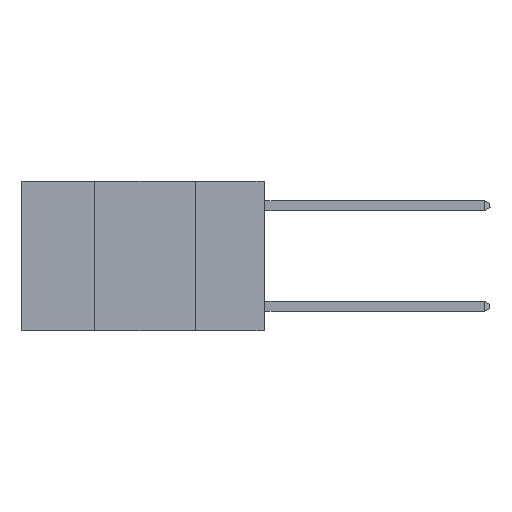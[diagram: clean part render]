
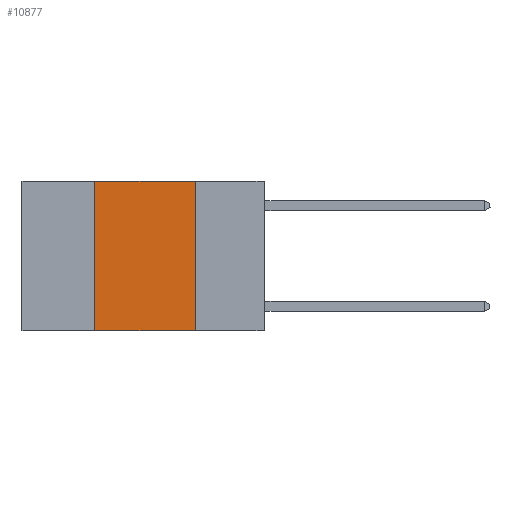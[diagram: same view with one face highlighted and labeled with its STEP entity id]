
A CAD part, left-side view. The second image highlights one B-rep face of the part: STEP entity #10877.
In plain terms, the highlighted planar face has unit normal (-1, 0, 0).
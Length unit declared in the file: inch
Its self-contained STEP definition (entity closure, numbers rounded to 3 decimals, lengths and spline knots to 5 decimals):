
#200 = AXIS2_PLACEMENT_3D ( 'NONE', #25338, #23256, #19574 ) ;
#3056 = CARTESIAN_POINT ( 'NONE',  ( 0., 0.17, 0. ) ) ;
#4137 = VECTOR ( 'NONE', #25794, 39.37008 ) ;
#4219 = CARTESIAN_POINT ( 'NONE',  ( 0., 0.6, 0. ) ) ;
#5190 = CARTESIAN_POINT ( 'NONE',  ( 0., 0.6, -0.37 ) ) ;
#5335 = LINE ( 'NONE', #5190, #27424 ) ;
#6482 = VERTEX_POINT ( 'NONE', #24693 ) ;
#6800 = CARTESIAN_POINT ( 'NONE',  ( 0., 0.42, 0. ) ) ;
#9617 = CARTESIAN_POINT ( 'NONE',  ( 0., 0.17, -0.37 ) ) ;
#9890 = EDGE_CURVE ( 'NONE', #15368, #20033, #17591, .T. ) ;
#10433 = DIRECTION ( 'NONE',  ( 0., 0., 1. ) ) ;
#10745 = EDGE_CURVE ( 'NONE', #6482, #15368, #25072, .T. ) ;
#10877 = ADVANCED_FACE ( 'NONE', ( #12530 ), #21025, .F. ) ;
#11447 = CARTESIAN_POINT ( 'NONE',  ( 0., 0.17, 0. ) ) ;
#12530 = FACE_OUTER_BOUND ( 'NONE', #26441, .T. ) ;
#12691 = VECTOR ( 'NONE', #10433, 39.37008 ) ;
#13400 = VERTEX_POINT ( 'NONE', #9617 ) ;
#14685 = ORIENTED_EDGE ( 'NONE', *, *, #10745, .F. ) ;
#15368 = VERTEX_POINT ( 'NONE', #6800 ) ;
#16486 = EDGE_CURVE ( 'NONE', #20033, #13400, #19671, .T. ) ;
#17591 = LINE ( 'NONE', #4219, #26394 ) ;
#17632 = CARTESIAN_POINT ( 'NONE',  ( 0., 0.42, 0. ) ) ;
#18047 = ORIENTED_EDGE ( 'NONE', *, *, #9890, .F. ) ;
#18813 = ORIENTED_EDGE ( 'NONE', *, *, #16486, .F. ) ;
#19574 = DIRECTION ( 'NONE',  ( 0., 0., -1. ) ) ;
#19671 = LINE ( 'NONE', #11447, #4137 ) ;
#20033 = VERTEX_POINT ( 'NONE', #3056 ) ;
#21025 = PLANE ( 'NONE',  #200 ) ;
#23256 = DIRECTION ( 'NONE',  ( 1., 0., 0. ) ) ;
#23675 = EDGE_CURVE ( 'NONE', #6482, #13400, #5335, .T. ) ;
#23852 = DIRECTION ( 'NONE',  ( 0., -1., 0. ) ) ;
#24567 = DIRECTION ( 'NONE',  ( 0., -1., 0. ) ) ;
#24636 = ORIENTED_EDGE ( 'NONE', *, *, #23675, .T. ) ;
#24693 = CARTESIAN_POINT ( 'NONE',  ( 0., 0.42, -0.37 ) ) ;
#25072 = LINE ( 'NONE', #17632, #12691 ) ;
#25338 = CARTESIAN_POINT ( 'NONE',  ( 0., 0.6, 0. ) ) ;
#25794 = DIRECTION ( 'NONE',  ( 0., 0., -1. ) ) ;
#26394 = VECTOR ( 'NONE', #23852, 39.37008 ) ;
#26441 = EDGE_LOOP ( 'NONE', ( #18813, #18047, #14685, #24636 ) ) ;
#27424 = VECTOR ( 'NONE', #24567, 39.37008 ) ;
